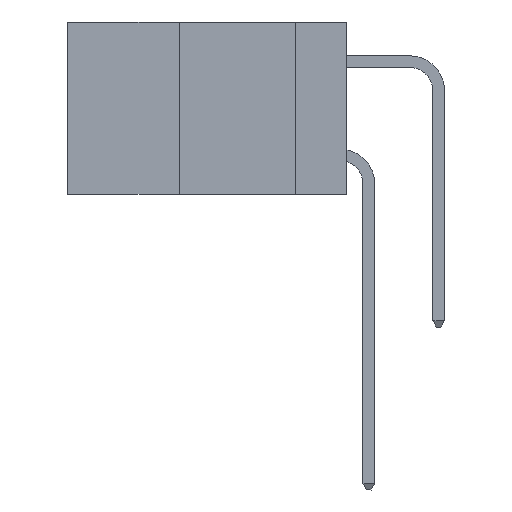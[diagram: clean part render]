
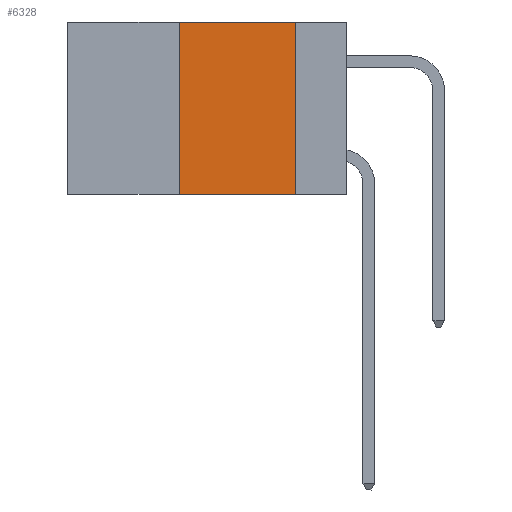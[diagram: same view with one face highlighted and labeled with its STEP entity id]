
A CAD part, left-side view. The second image highlights one B-rep face of the part: STEP entity #6328.
In plain terms, the highlighted planar face has unit normal (-1, 0, 0).
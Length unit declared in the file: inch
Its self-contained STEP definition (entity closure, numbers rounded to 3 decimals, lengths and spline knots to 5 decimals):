
#246 = EDGE_CURVE ( 'NONE', #10003, #260, #9413, .T. ) ;
#260 = VERTEX_POINT ( 'NONE', #1688 ) ;
#802 = CARTESIAN_POINT ( 'NONE',  ( 0., 0.6, -0.37 ) ) ;
#921 = ORIENTED_EDGE ( 'NONE', *, *, #9265, .F. ) ;
#1688 = CARTESIAN_POINT ( 'NONE',  ( 0., 0.11, 0. ) ) ;
#1727 = DIRECTION ( 'NONE',  ( 0., 0., 1. ) ) ;
#1844 = VERTEX_POINT ( 'NONE', #5555 ) ;
#2073 = VECTOR ( 'NONE', #6191, 39.37008 ) ;
#2613 = CARTESIAN_POINT ( 'NONE',  ( 0., 0.6, 0. ) ) ;
#3697 = ORIENTED_EDGE ( 'NONE', *, *, #246, .F. ) ;
#3741 = VERTEX_POINT ( 'NONE', #4607 ) ;
#4050 = VECTOR ( 'NONE', #7705, 39.37008 ) ;
#4390 = LINE ( 'NONE', #802, #4050 ) ;
#4590 = VECTOR ( 'NONE', #1727, 39.37008 ) ;
#4607 = CARTESIAN_POINT ( 'NONE',  ( 0., 0.36, -0.37 ) ) ;
#4648 = ORIENTED_EDGE ( 'NONE', *, *, #8716, .T. ) ;
#5002 = ORIENTED_EDGE ( 'NONE', *, *, #8552, .F. ) ;
#5351 = LINE ( 'NONE', #7270, #2073 ) ;
#5555 = CARTESIAN_POINT ( 'NONE',  ( 0., 0.11, -0.37 ) ) ;
#5776 = DIRECTION ( 'NONE',  ( 0., -1., 0. ) ) ;
#5965 = FACE_OUTER_BOUND ( 'NONE', #9468, .T. ) ;
#6024 = PLANE ( 'NONE',  #6158 ) ;
#6079 = DIRECTION ( 'NONE',  ( 1., 0., 0. ) ) ;
#6158 = AXIS2_PLACEMENT_3D ( 'NONE', #2613, #6079, #9432 ) ;
#6191 = DIRECTION ( 'NONE',  ( 0., 0., -1. ) ) ;
#6328 = ADVANCED_FACE ( 'NONE', ( #5965 ), #6024, .F. ) ;
#7064 = LINE ( 'NONE', #9620, #4590 ) ;
#7270 = CARTESIAN_POINT ( 'NONE',  ( 0., 0.11, 0. ) ) ;
#7705 = DIRECTION ( 'NONE',  ( 0., -1., 0. ) ) ;
#8552 = EDGE_CURVE ( 'NONE', #260, #1844, #5351, .T. ) ;
#8716 = EDGE_CURVE ( 'NONE', #3741, #1844, #4390, .T. ) ;
#9265 = EDGE_CURVE ( 'NONE', #3741, #10003, #7064, .T. ) ;
#9413 = LINE ( 'NONE', #11101, #10820 ) ;
#9432 = DIRECTION ( 'NONE',  ( 0., 0., -1. ) ) ;
#9468 = EDGE_LOOP ( 'NONE', ( #5002, #3697, #921, #4648 ) ) ;
#9620 = CARTESIAN_POINT ( 'NONE',  ( 0., 0.36, 0. ) ) ;
#10003 = VERTEX_POINT ( 'NONE', #10891 ) ;
#10820 = VECTOR ( 'NONE', #5776, 39.37008 ) ;
#10891 = CARTESIAN_POINT ( 'NONE',  ( 0., 0.36, 0. ) ) ;
#11101 = CARTESIAN_POINT ( 'NONE',  ( 0., 0.6, 0. ) ) ;
